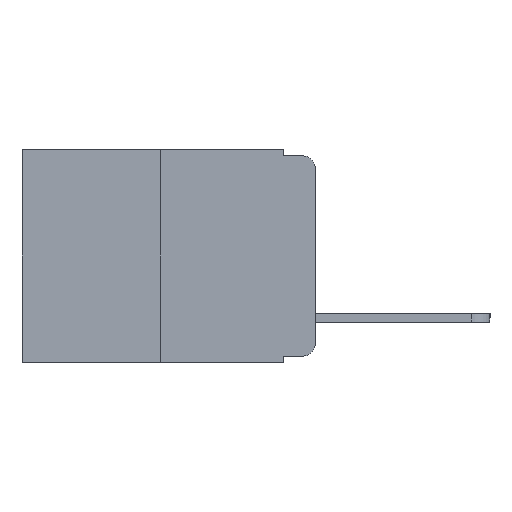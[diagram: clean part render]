
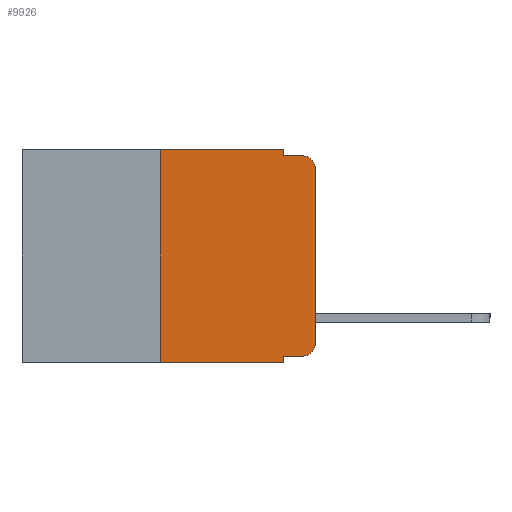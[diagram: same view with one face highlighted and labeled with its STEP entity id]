
A CAD part, left-side view. The second image highlights one B-rep face of the part: STEP entity #9926.
In plain terms, the highlighted planar face has unit normal (-1, 0, 0).
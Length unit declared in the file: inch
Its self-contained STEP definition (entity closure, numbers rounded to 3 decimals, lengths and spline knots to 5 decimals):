
#3 = VERTEX_POINT ( 'NONE', #122 ) ;
#59 = CARTESIAN_POINT ( 'NONE',  ( 0., 0.25, 0. ) ) ;
#122 = CARTESIAN_POINT ( 'NONE',  ( 0., 0.02, -0.333 ) ) ;
#229 = CARTESIAN_POINT ( 'NONE',  ( 0., 0.051, -0.343 ) ) ;
#298 = CARTESIAN_POINT ( 'NONE',  ( 0., 0.02, -0.313 ) ) ;
#468 = EDGE_CURVE ( 'NONE', #10777, #1136, #4502, .T. ) ;
#815 = CARTESIAN_POINT ( 'NONE',  ( 0., 0.051, -0.01 ) ) ;
#1136 = VERTEX_POINT ( 'NONE', #59 ) ;
#1154 = DIRECTION ( 'NONE',  ( 0., 0., -1. ) ) ;
#1284 = CIRCLE ( 'NONE', #1373, 0.02 ) ;
#1314 = EDGE_LOOP ( 'NONE', ( #2458, #6273, #8414, #13262, #9959, #2073, #3692, #12055, #6989, #4218 ) ) ;
#1342 = VECTOR ( 'NONE', #1748, 39.37008 ) ;
#1373 = AXIS2_PLACEMENT_3D ( 'NONE', #298, #5089, #11562 ) ;
#1508 = VERTEX_POINT ( 'NONE', #229 ) ;
#1560 = EDGE_CURVE ( 'NONE', #3, #9956, #1284, .T. ) ;
#1583 = CARTESIAN_POINT ( 'NONE',  ( 0., 0.051, 0. ) ) ;
#1692 = LINE ( 'NONE', #6643, #1342 ) ;
#1748 = DIRECTION ( 'NONE',  ( 0., 0., 1. ) ) ;
#1897 = EDGE_CURVE ( 'NONE', #10777, #1508, #11603, .T. ) ;
#1957 = CARTESIAN_POINT ( 'NONE',  ( 0., 0., -0.03 ) ) ;
#2019 = PLANE ( 'NONE',  #13793 ) ;
#2073 = ORIENTED_EDGE ( 'NONE', *, *, #468, .F. ) ;
#2222 = VECTOR ( 'NONE', #9847, 39.37008 ) ;
#2354 = LINE ( 'NONE', #6567, #11265 ) ;
#2458 = ORIENTED_EDGE ( 'NONE', *, *, #5996, .T. ) ;
#2811 = EDGE_CURVE ( 'NONE', #7014, #5851, #2354, .T. ) ;
#3027 = CARTESIAN_POINT ( 'NONE',  ( 0., 0.25, 0. ) ) ;
#3175 = DIRECTION ( 'NONE',  ( 1., 0., 0. ) ) ;
#3423 = DIRECTION ( 'NONE',  ( 0., -1., 0. ) ) ;
#3645 = CARTESIAN_POINT ( 'NONE',  ( 0., 0.473, 0. ) ) ;
#3692 = ORIENTED_EDGE ( 'NONE', *, *, #1897, .T. ) ;
#4041 = DIRECTION ( 'NONE',  ( 0., -1., 0. ) ) ;
#4154 = VECTOR ( 'NONE', #8894, 39.37008 ) ;
#4218 = ORIENTED_EDGE ( 'NONE', *, *, #1560, .T. ) ;
#4502 = LINE ( 'NONE', #3027, #4154 ) ;
#4542 = EDGE_CURVE ( 'NONE', #7291, #4780, #4573, .T. ) ;
#4573 = CIRCLE ( 'NONE', #7908, 0.02 ) ;
#4780 = VERTEX_POINT ( 'NONE', #12807 ) ;
#5089 = DIRECTION ( 'NONE',  ( -1., 0., 0. ) ) ;
#5185 = LINE ( 'NONE', #9800, #2222 ) ;
#5193 = CARTESIAN_POINT ( 'NONE',  ( 0., 0.051, -0.01 ) ) ;
#5376 = CARTESIAN_POINT ( 'NONE',  ( 0., 0., -0.313 ) ) ;
#5526 = VERTEX_POINT ( 'NONE', #13422 ) ;
#5770 = EDGE_CURVE ( 'NONE', #5851, #4780, #7503, .T. ) ;
#5851 = VERTEX_POINT ( 'NONE', #5193 ) ;
#5949 = CARTESIAN_POINT ( 'NONE',  ( 0., 0.25, -0.343 ) ) ;
#5996 = EDGE_CURVE ( 'NONE', #9956, #7291, #1692, .T. ) ;
#6273 = ORIENTED_EDGE ( 'NONE', *, *, #4542, .T. ) ;
#6373 = CARTESIAN_POINT ( 'NONE',  ( 0., 0.473, -0.343 ) ) ;
#6407 = CARTESIAN_POINT ( 'NONE',  ( 0., 0.473, 0. ) ) ;
#6567 = CARTESIAN_POINT ( 'NONE',  ( 0., 0.051, 0. ) ) ;
#6643 = CARTESIAN_POINT ( 'NONE',  ( 0., 0., 0. ) ) ;
#6989 = ORIENTED_EDGE ( 'NONE', *, *, #12326, .T. ) ;
#7014 = VERTEX_POINT ( 'NONE', #1583 ) ;
#7291 = VERTEX_POINT ( 'NONE', #1957 ) ;
#7503 = LINE ( 'NONE', #815, #10478 ) ;
#7702 = DIRECTION ( 'NONE',  ( 0., 0., -1. ) ) ;
#7908 = AXIS2_PLACEMENT_3D ( 'NONE', #9585, #9560, #1154 ) ;
#8268 = LINE ( 'NONE', #3645, #10535 ) ;
#8414 = ORIENTED_EDGE ( 'NONE', *, *, #5770, .F. ) ;
#8635 = VECTOR ( 'NONE', #4041, 39.37008 ) ;
#8894 = DIRECTION ( 'NONE',  ( 0., 0., 1. ) ) ;
#8975 = CARTESIAN_POINT ( 'NONE',  ( 0., 0.051, -0.333 ) ) ;
#9248 = LINE ( 'NONE', #8975, #14423 ) ;
#9433 = DIRECTION ( 'NONE',  ( 0., -1., 0. ) ) ;
#9527 = EDGE_CURVE ( 'NONE', #1136, #7014, #8268, .T. ) ;
#9560 = DIRECTION ( 'NONE',  ( -1., 0., 0. ) ) ;
#9585 = CARTESIAN_POINT ( 'NONE',  ( 0., 0.02, -0.03 ) ) ;
#9800 = CARTESIAN_POINT ( 'NONE',  ( 0., 0.051, 0. ) ) ;
#9847 = DIRECTION ( 'NONE',  ( 0., 0., -1. ) ) ;
#9926 = ADVANCED_FACE ( 'NONE', ( #11560 ), #2019, .F. ) ;
#9956 = VERTEX_POINT ( 'NONE', #5376 ) ;
#9959 = ORIENTED_EDGE ( 'NONE', *, *, #9527, .F. ) ;
#10478 = VECTOR ( 'NONE', #9433, 39.37008 ) ;
#10535 = VECTOR ( 'NONE', #12525, 39.37008 ) ;
#10777 = VERTEX_POINT ( 'NONE', #5949 ) ;
#10996 = DIRECTION ( 'NONE',  ( 0., 0., -1. ) ) ;
#11265 = VECTOR ( 'NONE', #7702, 39.37008 ) ;
#11560 = FACE_OUTER_BOUND ( 'NONE', #1314, .T. ) ;
#11562 = DIRECTION ( 'NONE',  ( 0., 0., -1. ) ) ;
#11603 = LINE ( 'NONE', #6373, #8635 ) ;
#12055 = ORIENTED_EDGE ( 'NONE', *, *, #12799, .F. ) ;
#12326 = EDGE_CURVE ( 'NONE', #5526, #3, #9248, .T. ) ;
#12525 = DIRECTION ( 'NONE',  ( 0., -1., 0. ) ) ;
#12799 = EDGE_CURVE ( 'NONE', #5526, #1508, #5185, .T. ) ;
#12807 = CARTESIAN_POINT ( 'NONE',  ( 0., 0.02, -0.01 ) ) ;
#13262 = ORIENTED_EDGE ( 'NONE', *, *, #2811, .F. ) ;
#13422 = CARTESIAN_POINT ( 'NONE',  ( 0., 0.051, -0.333 ) ) ;
#13793 = AXIS2_PLACEMENT_3D ( 'NONE', #6407, #3175, #10996 ) ;
#14423 = VECTOR ( 'NONE', #3423, 39.37008 ) ;
